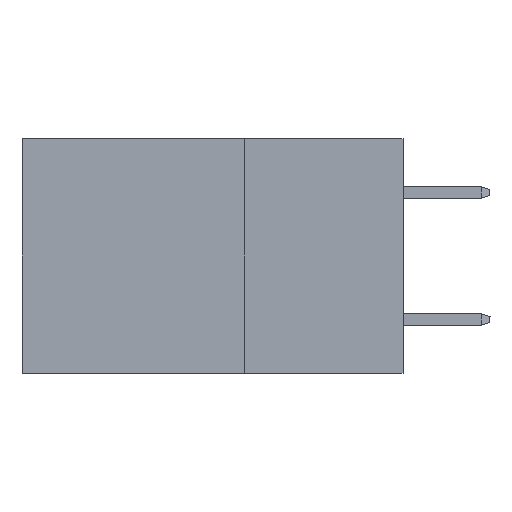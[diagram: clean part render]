
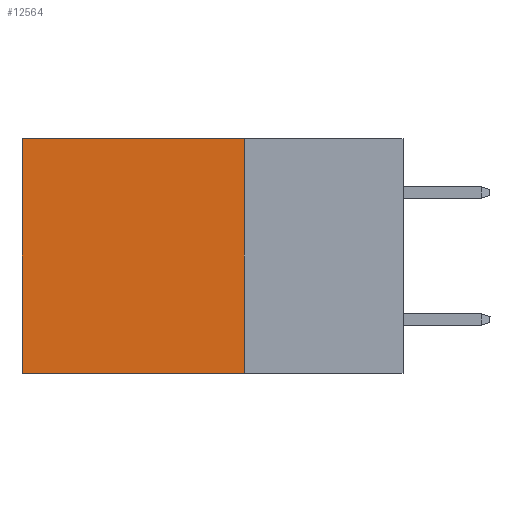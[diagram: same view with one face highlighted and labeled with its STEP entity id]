
A CAD part, left-side view. The second image highlights one B-rep face of the part: STEP entity #12564.
In plain terms, the highlighted planar face has unit normal (-1, 0, 0).
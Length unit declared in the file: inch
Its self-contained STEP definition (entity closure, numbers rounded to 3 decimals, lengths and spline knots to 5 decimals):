
#972 = VERTEX_POINT ( 'NONE', #2527 ) ;
#1685 = CARTESIAN_POINT ( 'NONE',  ( 0.2875, 0.25, 0. ) ) ;
#2527 = CARTESIAN_POINT ( 'NONE',  ( 0.2875, 0.6, 0. ) ) ;
#3335 = VERTEX_POINT ( 'NONE', #35899 ) ;
#3364 = ORIENTED_EDGE ( 'NONE', *, *, #18785, .T. ) ;
#4002 = CARTESIAN_POINT ( 'NONE',  ( 0.2875, 0.25, 0. ) ) ;
#5648 = DIRECTION ( 'NONE',  ( 0., 1., 0. ) ) ;
#6715 = PLANE ( 'NONE',  #32212 ) ;
#7015 = VERTEX_POINT ( 'NONE', #7762 ) ;
#7762 = CARTESIAN_POINT ( 'NONE',  ( 0.2875, 0.25, 0. ) ) ;
#8077 = LINE ( 'NONE', #33299, #11465 ) ;
#9669 = EDGE_CURVE ( 'NONE', #7015, #972, #33326, .T. ) ;
#11465 = VECTOR ( 'NONE', #40115, 39.37008 ) ;
#12564 = ADVANCED_FACE ( 'NONE', ( #19903 ), #6715, .F. ) ;
#14552 = VECTOR ( 'NONE', #20908, 39.37008 ) ;
#17307 = ORIENTED_EDGE ( 'NONE', *, *, #33401, .F. ) ;
#18623 = LINE ( 'NONE', #30859, #14552 ) ;
#18785 = EDGE_CURVE ( 'NONE', #972, #3335, #8077, .T. ) ;
#19723 = EDGE_LOOP ( 'NONE', ( #3364, #34110, #17307, #37645 ) ) ;
#19903 = FACE_OUTER_BOUND ( 'NONE', #19723, .T. ) ;
#20310 = EDGE_CURVE ( 'NONE', #31006, #3335, #33977, .T. ) ;
#20693 = VECTOR ( 'NONE', #5648, 39.37008 ) ;
#20792 = CARTESIAN_POINT ( 'NONE',  ( 0.2875, 0.25, -0.37 ) ) ;
#20908 = DIRECTION ( 'NONE',  ( 0., 0., -1. ) ) ;
#22424 = DIRECTION ( 'NONE',  ( 1., 0., 0. ) ) ;
#24227 = DIRECTION ( 'NONE',  ( 0., 1., 0. ) ) ;
#30859 = CARTESIAN_POINT ( 'NONE',  ( 0.2875, 0.25, 0. ) ) ;
#31006 = VERTEX_POINT ( 'NONE', #20792 ) ;
#32212 = AXIS2_PLACEMENT_3D ( 'NONE', #4002, #22424, #35235 ) ;
#33299 = CARTESIAN_POINT ( 'NONE',  ( 0.2875, 0.6, 0. ) ) ;
#33326 = LINE ( 'NONE', #1685, #35823 ) ;
#33401 = EDGE_CURVE ( 'NONE', #7015, #31006, #18623, .T. ) ;
#33977 = LINE ( 'NONE', #37707, #20693 ) ;
#34110 = ORIENTED_EDGE ( 'NONE', *, *, #20310, .F. ) ;
#35235 = DIRECTION ( 'NONE',  ( 0., 0., -1. ) ) ;
#35823 = VECTOR ( 'NONE', #24227, 39.37008 ) ;
#35899 = CARTESIAN_POINT ( 'NONE',  ( 0.2875, 0.6, -0.37 ) ) ;
#37645 = ORIENTED_EDGE ( 'NONE', *, *, #9669, .T. ) ;
#37707 = CARTESIAN_POINT ( 'NONE',  ( 0.2875, 0.25, -0.37 ) ) ;
#40115 = DIRECTION ( 'NONE',  ( 0., 0., -1. ) ) ;
